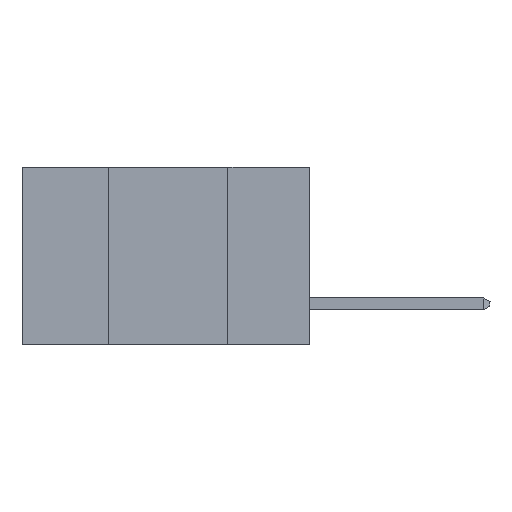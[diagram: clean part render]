
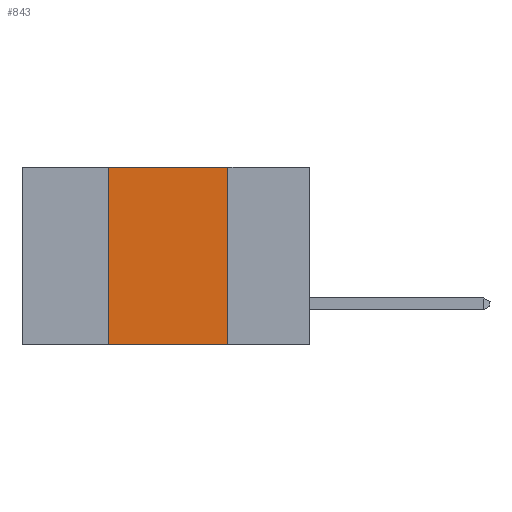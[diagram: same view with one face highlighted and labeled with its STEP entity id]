
A CAD part, left-side view. The second image highlights one B-rep face of the part: STEP entity #843.
In plain terms, the highlighted planar face has unit normal (-1, 0, 0).
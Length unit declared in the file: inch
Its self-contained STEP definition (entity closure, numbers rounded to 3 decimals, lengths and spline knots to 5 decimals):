
#843 = ADVANCED_FACE ( 'NONE', ( #18839 ), #13894, .F. ) ;
#2784 = LINE ( 'NONE', #8111, #33687 ) ;
#3714 = VECTOR ( 'NONE', #38531, 39.37008 ) ;
#4125 = LINE ( 'NONE', #9853, #30228 ) ;
#5788 = CARTESIAN_POINT ( 'NONE',  ( 0., 0.6, -0.37 ) ) ;
#7200 = DIRECTION ( 'NONE',  ( 1., 0., 0. ) ) ;
#8025 = VERTEX_POINT ( 'NONE', #20542 ) ;
#8111 = CARTESIAN_POINT ( 'NONE',  ( 0., 0.17, 0. ) ) ;
#8610 = VERTEX_POINT ( 'NONE', #21272 ) ;
#9853 = CARTESIAN_POINT ( 'NONE',  ( 0., 0.42, 0. ) ) ;
#11456 = AXIS2_PLACEMENT_3D ( 'NONE', #19608, #7200, #16267 ) ;
#12423 = EDGE_CURVE ( 'NONE', #8610, #17794, #2784, .T. ) ;
#12500 = CARTESIAN_POINT ( 'NONE',  ( 0., 0.42, -0.37 ) ) ;
#13894 = PLANE ( 'NONE',  #11456 ) ;
#15054 = LINE ( 'NONE', #5788, #3714 ) ;
#16267 = DIRECTION ( 'NONE',  ( 0., 0., -1. ) ) ;
#17081 = CARTESIAN_POINT ( 'NONE',  ( 0., 0.6, 0. ) ) ;
#17794 = VERTEX_POINT ( 'NONE', #28487 ) ;
#18839 = FACE_OUTER_BOUND ( 'NONE', #28923, .T. ) ;
#19407 = VERTEX_POINT ( 'NONE', #12500 ) ;
#19608 = CARTESIAN_POINT ( 'NONE',  ( 0., 0.6, 0. ) ) ;
#20542 = CARTESIAN_POINT ( 'NONE',  ( 0., 0.42, 0. ) ) ;
#20904 = ORIENTED_EDGE ( 'NONE', *, *, #34816, .T. ) ;
#21272 = CARTESIAN_POINT ( 'NONE',  ( 0., 0.17, 0. ) ) ;
#26081 = ORIENTED_EDGE ( 'NONE', *, *, #28073, .F. ) ;
#28073 = EDGE_CURVE ( 'NONE', #8025, #8610, #37791, .T. ) ;
#28487 = CARTESIAN_POINT ( 'NONE',  ( 0., 0.17, -0.37 ) ) ;
#28846 = EDGE_CURVE ( 'NONE', #19407, #8025, #4125, .T. ) ;
#28923 = EDGE_LOOP ( 'NONE', ( #38099, #26081, #34545, #20904 ) ) ;
#29400 = DIRECTION ( 'NONE',  ( 0., 0., -1. ) ) ;
#30228 = VECTOR ( 'NONE', #37073, 39.37008 ) ;
#30867 = VECTOR ( 'NONE', #34819, 39.37008 ) ;
#33687 = VECTOR ( 'NONE', #29400, 39.37008 ) ;
#34545 = ORIENTED_EDGE ( 'NONE', *, *, #28846, .F. ) ;
#34816 = EDGE_CURVE ( 'NONE', #19407, #17794, #15054, .T. ) ;
#34819 = DIRECTION ( 'NONE',  ( 0., -1., 0. ) ) ;
#37073 = DIRECTION ( 'NONE',  ( 0., 0., 1. ) ) ;
#37791 = LINE ( 'NONE', #17081, #30867 ) ;
#38099 = ORIENTED_EDGE ( 'NONE', *, *, #12423, .F. ) ;
#38531 = DIRECTION ( 'NONE',  ( 0., -1., 0. ) ) ;
